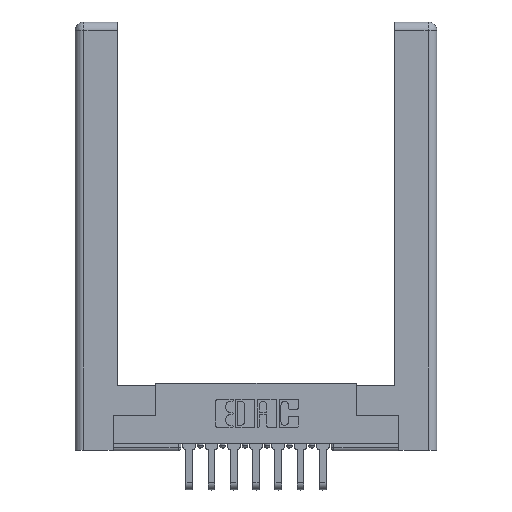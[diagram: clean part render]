
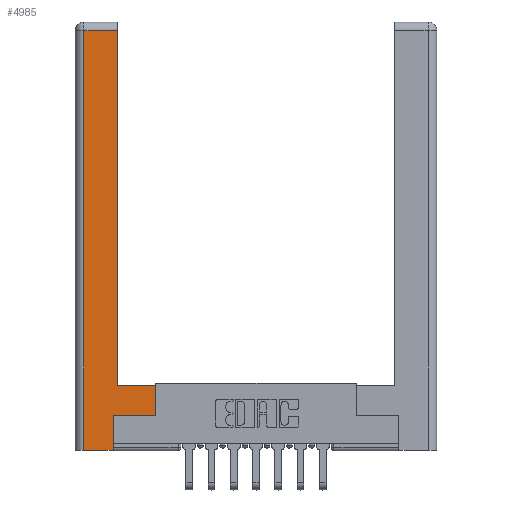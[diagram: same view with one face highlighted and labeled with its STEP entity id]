
A CAD part, top view. The second image highlights one B-rep face of the part: STEP entity #4985.
In plain terms, the highlighted planar face has unit normal (0, 0, 1).
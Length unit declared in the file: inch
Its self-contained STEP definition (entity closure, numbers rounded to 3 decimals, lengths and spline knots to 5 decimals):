
#6 = CARTESIAN_POINT ( 'NONE',  ( 0.565, 0.245, 0. ) ) ;
#182 = LINE ( 'NONE', #9119, #6484 ) ;
#251 = VERTEX_POINT ( 'NONE', #12687 ) ;
#423 = DIRECTION ( 'NONE',  ( -1., 0., 0. ) ) ;
#461 = EDGE_CURVE ( 'NONE', #2699, #3797, #182, .T. ) ;
#936 = LINE ( 'NONE', #3251, #4077 ) ;
#977 = DIRECTION ( 'NONE',  ( 0., -1., 0. ) ) ;
#1269 = PLANE ( 'NONE',  #8087 ) ;
#1275 = LINE ( 'NONE', #12106, #6938 ) ;
#1655 = CARTESIAN_POINT ( 'NONE',  ( 0.265, 0., 0. ) ) ;
#1916 = CARTESIAN_POINT ( 'NONE',  ( 0.265, 0.245, 0. ) ) ;
#2134 = ORIENTED_EDGE ( 'NONE', *, *, #3799, .T. ) ;
#2431 = CARTESIAN_POINT ( 'NONE',  ( 0.0615, 2.94, 0. ) ) ;
#2444 = ORIENTED_EDGE ( 'NONE', *, *, #12238, .T. ) ;
#2699 = VERTEX_POINT ( 'NONE', #10473 ) ;
#2869 = ORIENTED_EDGE ( 'NONE', *, *, #2884, .T. ) ;
#2884 = EDGE_CURVE ( 'NONE', #11421, #12749, #5708, .T. ) ;
#3049 = CARTESIAN_POINT ( 'NONE',  ( 0.0615, 0., 0. ) ) ;
#3171 = VECTOR ( 'NONE', #12842, 39.37008 ) ;
#3251 = CARTESIAN_POINT ( 'NONE',  ( 0.295, 3., 0. ) ) ;
#3364 = DIRECTION ( 'NONE',  ( 0., 0., -1. ) ) ;
#3633 = FACE_OUTER_BOUND ( 'NONE', #7907, .T. ) ;
#3712 = VECTOR ( 'NONE', #12059, 39.37008 ) ;
#3746 = CARTESIAN_POINT ( 'NONE',  ( 0.565, 0.45, 0. ) ) ;
#3797 = VERTEX_POINT ( 'NONE', #2431 ) ;
#3799 = EDGE_CURVE ( 'NONE', #12479, #251, #5085, .T. ) ;
#4077 = VECTOR ( 'NONE', #7342, 39.37008 ) ;
#4439 = LINE ( 'NONE', #7977, #6673 ) ;
#4985 = ADVANCED_FACE ( 'NONE', ( #3633 ), #1269, .F. ) ;
#5085 = LINE ( 'NONE', #5469, #9836 ) ;
#5469 = CARTESIAN_POINT ( 'NONE',  ( 0.295, 0.45, 0. ) ) ;
#5700 = DIRECTION ( 'NONE',  ( 1., 0., 0. ) ) ;
#5708 = LINE ( 'NONE', #1655, #3171 ) ;
#6096 = CARTESIAN_POINT ( 'NONE',  ( 0.265, 0.245, 0. ) ) ;
#6109 = DIRECTION ( 'NONE',  ( 0., 1., 0. ) ) ;
#6214 = ORIENTED_EDGE ( 'NONE', *, *, #11431, .T. ) ;
#6419 = LINE ( 'NONE', #1916, #3712 ) ;
#6484 = VECTOR ( 'NONE', #6557, 39.37008 ) ;
#6557 = DIRECTION ( 'NONE',  ( -1., 0., 0. ) ) ;
#6651 = ORIENTED_EDGE ( 'NONE', *, *, #10285, .T. ) ;
#6673 = VECTOR ( 'NONE', #977, 39.37008 ) ;
#6938 = VECTOR ( 'NONE', #6109, 39.37008 ) ;
#6996 = VERTEX_POINT ( 'NONE', #6 ) ;
#7342 = DIRECTION ( 'NONE',  ( 0., 1., 0. ) ) ;
#7907 = EDGE_LOOP ( 'NONE', ( #2444, #8115, #6651, #2869, #8882, #8510, #6214, #2134 ) ) ;
#7960 = EDGE_CURVE ( 'NONE', #12014, #6996, #10856, .T. ) ;
#7977 = CARTESIAN_POINT ( 'NONE',  ( 0.0615, 0., 0. ) ) ;
#8087 = AXIS2_PLACEMENT_3D ( 'NONE', #10431, #3364, #423 ) ;
#8115 = ORIENTED_EDGE ( 'NONE', *, *, #461, .T. ) ;
#8250 = EDGE_CURVE ( 'NONE', #12749, #12014, #6419, .T. ) ;
#8510 = ORIENTED_EDGE ( 'NONE', *, *, #7960, .T. ) ;
#8522 = CARTESIAN_POINT ( 'NONE',  ( 0.565, 0.245, 0. ) ) ;
#8882 = ORIENTED_EDGE ( 'NONE', *, *, #8250, .T. ) ;
#8921 = CARTESIAN_POINT ( 'NONE',  ( 0.265, 0., 0. ) ) ;
#9119 = CARTESIAN_POINT ( 'NONE',  ( 0.0615, 2.94, 0. ) ) ;
#9580 = DIRECTION ( 'NONE',  ( -1., 0., 0. ) ) ;
#9836 = VECTOR ( 'NONE', #9580, 39.37008 ) ;
#10285 = EDGE_CURVE ( 'NONE', #3797, #11421, #4439, .T. ) ;
#10431 = CARTESIAN_POINT ( 'NONE',  ( 0., 0., 0. ) ) ;
#10473 = CARTESIAN_POINT ( 'NONE',  ( 0.295, 2.94, 0. ) ) ;
#10856 = LINE ( 'NONE', #8522, #11638 ) ;
#11421 = VERTEX_POINT ( 'NONE', #3049 ) ;
#11431 = EDGE_CURVE ( 'NONE', #6996, #12479, #1275, .T. ) ;
#11638 = VECTOR ( 'NONE', #5700, 39.37008 ) ;
#12014 = VERTEX_POINT ( 'NONE', #6096 ) ;
#12059 = DIRECTION ( 'NONE',  ( 0., 1., 0. ) ) ;
#12106 = CARTESIAN_POINT ( 'NONE',  ( 0.565, 0.45, 0. ) ) ;
#12238 = EDGE_CURVE ( 'NONE', #251, #2699, #936, .T. ) ;
#12479 = VERTEX_POINT ( 'NONE', #3746 ) ;
#12687 = CARTESIAN_POINT ( 'NONE',  ( 0.295, 0.45, 0. ) ) ;
#12749 = VERTEX_POINT ( 'NONE', #8921 ) ;
#12842 = DIRECTION ( 'NONE',  ( 1., 0., 0. ) ) ;
